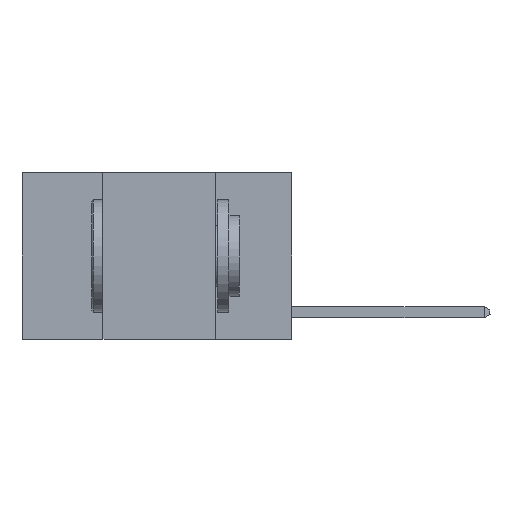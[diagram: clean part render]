
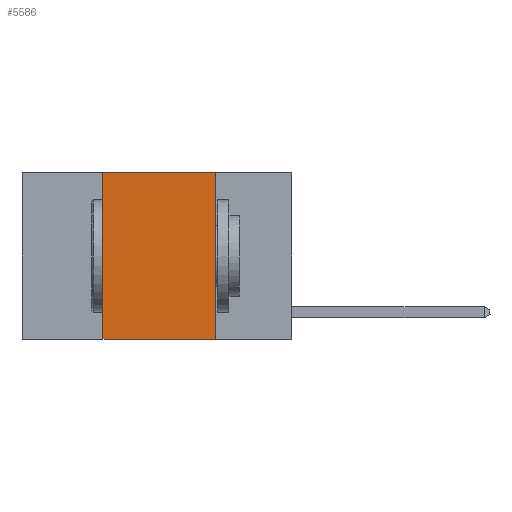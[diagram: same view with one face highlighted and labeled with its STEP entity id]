
A CAD part, left-side view. The second image highlights one B-rep face of the part: STEP entity #5586.
In plain terms, the highlighted planar face has unit normal (-1, 0, 0).
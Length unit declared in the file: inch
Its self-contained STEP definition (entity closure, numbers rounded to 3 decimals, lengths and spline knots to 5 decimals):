
#212 = CARTESIAN_POINT ( 'NONE',  ( 0., 0.6, -0.37 ) ) ;
#218 = EDGE_CURVE ( 'NONE', #2293, #9196, #2559, .T. ) ;
#953 = DIRECTION ( 'NONE',  ( 0., -1., 0. ) ) ;
#964 = VERTEX_POINT ( 'NONE', #4093 ) ;
#1175 = DIRECTION ( 'NONE',  ( 0., 0., 1. ) ) ;
#1184 = VECTOR ( 'NONE', #1175, 39.37008 ) ;
#1507 = EDGE_CURVE ( 'NONE', #7952, #964, #6987, .T. ) ;
#2293 = VERTEX_POINT ( 'NONE', #6732 ) ;
#2559 = LINE ( 'NONE', #212, #5555 ) ;
#2959 = CARTESIAN_POINT ( 'NONE',  ( 0., 0.42, 0. ) ) ;
#3637 = EDGE_CURVE ( 'NONE', #964, #9196, #4165, .T. ) ;
#3701 = PLANE ( 'NONE',  #7899 ) ;
#3771 = DIRECTION ( 'NONE',  ( 0., 0., -1. ) ) ;
#3834 = LINE ( 'NONE', #2959, #1184 ) ;
#4093 = CARTESIAN_POINT ( 'NONE',  ( 0., 0.17, 0. ) ) ;
#4165 = LINE ( 'NONE', #10247, #5013 ) ;
#4896 = ORIENTED_EDGE ( 'NONE', *, *, #1507, .F. ) ;
#5013 = VECTOR ( 'NONE', #6787, 39.37008 ) ;
#5180 = EDGE_CURVE ( 'NONE', #2293, #7952, #3834, .T. ) ;
#5480 = CARTESIAN_POINT ( 'NONE',  ( 0., 0.6, 0. ) ) ;
#5555 = VECTOR ( 'NONE', #10478, 39.37008 ) ;
#5586 = ADVANCED_FACE ( 'NONE', ( #7256 ), #3701, .F. ) ;
#6104 = ORIENTED_EDGE ( 'NONE', *, *, #3637, .F. ) ;
#6283 = DIRECTION ( 'NONE',  ( 1., 0., 0. ) ) ;
#6732 = CARTESIAN_POINT ( 'NONE',  ( 0., 0.42, -0.37 ) ) ;
#6787 = DIRECTION ( 'NONE',  ( 0., 0., -1. ) ) ;
#6987 = LINE ( 'NONE', #7096, #7473 ) ;
#7088 = ORIENTED_EDGE ( 'NONE', *, *, #5180, .F. ) ;
#7096 = CARTESIAN_POINT ( 'NONE',  ( 0., 0.6, 0. ) ) ;
#7127 = ORIENTED_EDGE ( 'NONE', *, *, #218, .T. ) ;
#7144 = CARTESIAN_POINT ( 'NONE',  ( 0., 0.17, -0.37 ) ) ;
#7256 = FACE_OUTER_BOUND ( 'NONE', #9666, .T. ) ;
#7473 = VECTOR ( 'NONE', #953, 39.37008 ) ;
#7899 = AXIS2_PLACEMENT_3D ( 'NONE', #5480, #6283, #3771 ) ;
#7952 = VERTEX_POINT ( 'NONE', #10255 ) ;
#9196 = VERTEX_POINT ( 'NONE', #7144 ) ;
#9666 = EDGE_LOOP ( 'NONE', ( #6104, #4896, #7088, #7127 ) ) ;
#10247 = CARTESIAN_POINT ( 'NONE',  ( 0., 0.17, 0. ) ) ;
#10255 = CARTESIAN_POINT ( 'NONE',  ( 0., 0.42, 0. ) ) ;
#10478 = DIRECTION ( 'NONE',  ( 0., -1., 0. ) ) ;
